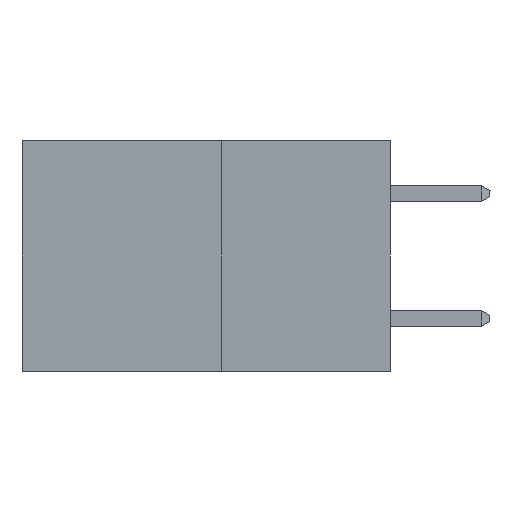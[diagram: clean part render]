
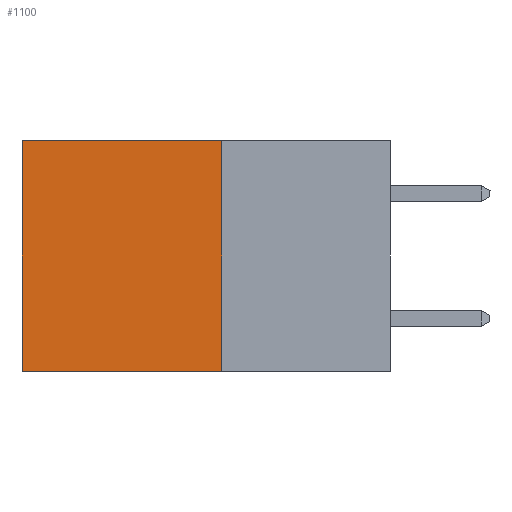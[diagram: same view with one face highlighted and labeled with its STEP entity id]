
A CAD part, left-side view. The second image highlights one B-rep face of the part: STEP entity #1100.
In plain terms, the highlighted planar face has unit normal (-1, 0, 0).
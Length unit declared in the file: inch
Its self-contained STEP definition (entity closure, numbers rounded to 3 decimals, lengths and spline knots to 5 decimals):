
#69 = CARTESIAN_POINT ( 'NONE',  ( 0.277, 0.59, -0.37 ) ) ;
#246 = EDGE_CURVE ( 'NONE', #3129, #8697, #5263, .T. ) ;
#263 = CARTESIAN_POINT ( 'NONE',  ( 0.277, 0.27, 0. ) ) ;
#478 = DIRECTION ( 'NONE',  ( 0., 0., -1. ) ) ;
#593 = ORIENTED_EDGE ( 'NONE', *, *, #8025, .T. ) ;
#970 = CARTESIAN_POINT ( 'NONE',  ( 0.277, 0.27, -0.37 ) ) ;
#1011 = DIRECTION ( 'NONE',  ( 0., 1., 0. ) ) ;
#1100 = ADVANCED_FACE ( 'NONE', ( #1394 ), #1237, .F. ) ;
#1137 = VECTOR ( 'NONE', #7332, 39.37008 ) ;
#1237 = PLANE ( 'NONE',  #1261 ) ;
#1238 = CARTESIAN_POINT ( 'NONE',  ( 0.277, 0.27, -0.37 ) ) ;
#1261 = AXIS2_PLACEMENT_3D ( 'NONE', #7435, #5537, #478 ) ;
#1394 = FACE_OUTER_BOUND ( 'NONE', #5555, .T. ) ;
#1581 = CARTESIAN_POINT ( 'NONE',  ( 0.277, 0.27, -0.37 ) ) ;
#2093 = ORIENTED_EDGE ( 'NONE', *, *, #6063, .T. ) ;
#3069 = ORIENTED_EDGE ( 'NONE', *, *, #246, .F. ) ;
#3129 = VERTEX_POINT ( 'NONE', #970 ) ;
#3157 = LINE ( 'NONE', #3302, #1137 ) ;
#3302 = CARTESIAN_POINT ( 'NONE',  ( 0.277, 0.59, -0.37 ) ) ;
#3361 = CARTESIAN_POINT ( 'NONE',  ( 0.277, 0.27, 0. ) ) ;
#3530 = DIRECTION ( 'NONE',  ( 0., 0., -1. ) ) ;
#3652 = VECTOR ( 'NONE', #4375, 39.37008 ) ;
#4065 = EDGE_CURVE ( 'NONE', #5252, #3129, #8325, .T. ) ;
#4116 = VECTOR ( 'NONE', #1011, 39.37008 ) ;
#4344 = LINE ( 'NONE', #3361, #4116 ) ;
#4375 = DIRECTION ( 'NONE',  ( 0., 1., 0. ) ) ;
#4437 = VERTEX_POINT ( 'NONE', #7069 ) ;
#4634 = ORIENTED_EDGE ( 'NONE', *, *, #4065, .F. ) ;
#5252 = VERTEX_POINT ( 'NONE', #263 ) ;
#5263 = LINE ( 'NONE', #1581, #3652 ) ;
#5537 = DIRECTION ( 'NONE',  ( 1., 0., 0. ) ) ;
#5555 = EDGE_LOOP ( 'NONE', ( #2093, #3069, #4634, #593 ) ) ;
#6063 = EDGE_CURVE ( 'NONE', #4437, #8697, #3157, .T. ) ;
#7069 = CARTESIAN_POINT ( 'NONE',  ( 0.277, 0.59, 0. ) ) ;
#7332 = DIRECTION ( 'NONE',  ( 0., 0., -1. ) ) ;
#7435 = CARTESIAN_POINT ( 'NONE',  ( 0.277, 0.27, -0.37 ) ) ;
#7908 = VECTOR ( 'NONE', #3530, 39.37008 ) ;
#8025 = EDGE_CURVE ( 'NONE', #5252, #4437, #4344, .T. ) ;
#8325 = LINE ( 'NONE', #1238, #7908 ) ;
#8697 = VERTEX_POINT ( 'NONE', #69 ) ;
